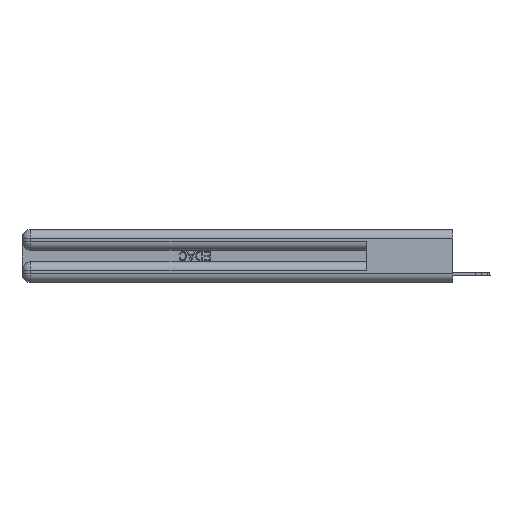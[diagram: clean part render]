
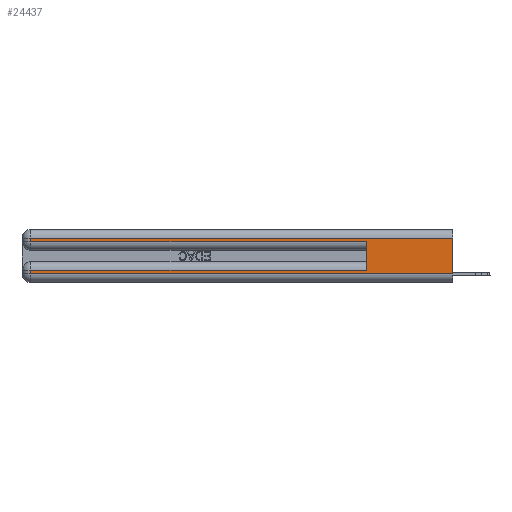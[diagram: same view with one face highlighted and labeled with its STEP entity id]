
A CAD part, left-side view. The second image highlights one B-rep face of the part: STEP entity #24437.
In plain terms, the highlighted planar face has unit normal (-1, 0, 0).
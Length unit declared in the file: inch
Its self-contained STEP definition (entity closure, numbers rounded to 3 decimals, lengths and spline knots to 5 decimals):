
#738 = EDGE_CURVE ( 'NONE', #1141, #9404, #14816, .T. ) ;
#751 = DIRECTION ( 'NONE',  ( 0., 0., -1. ) ) ;
#999 = LINE ( 'NONE', #17938, #28535 ) ;
#1023 = ORIENTED_EDGE ( 'NONE', *, *, #23884, .T. ) ;
#1141 = VERTEX_POINT ( 'NONE', #7086 ) ;
#3036 = LINE ( 'NONE', #12337, #10934 ) ;
#3364 = VECTOR ( 'NONE', #19117, 39.37008 ) ;
#3694 = ORIENTED_EDGE ( 'NONE', *, *, #4199, .T. ) ;
#4199 = EDGE_CURVE ( 'NONE', #7396, #12681, #21304, .T. ) ;
#4315 = VERTEX_POINT ( 'NONE', #29066 ) ;
#4872 = PLANE ( 'NONE',  #8600 ) ;
#5170 = VECTOR ( 'NONE', #24261, 39.37008 ) ;
#5258 = DIRECTION ( 'NONE',  ( 0., 1., 0. ) ) ;
#5300 = DIRECTION ( 'NONE',  ( 0., -1., 0. ) ) ;
#5316 = DIRECTION ( 'NONE',  ( 0., 0., -1. ) ) ;
#5409 = CARTESIAN_POINT ( 'NONE',  ( 0., 0., 0.085 ) ) ;
#6192 = EDGE_CURVE ( 'NONE', #12681, #4315, #3036, .T. ) ;
#7086 = CARTESIAN_POINT ( 'NONE',  ( 0., 0., 0.31 ) ) ;
#7396 = VERTEX_POINT ( 'NONE', #23852 ) ;
#8534 = VECTOR ( 'NONE', #5300, 39.37008 ) ;
#8600 = AXIS2_PLACEMENT_3D ( 'NONE', #16933, #12188, #5316 ) ;
#8640 = DIRECTION ( 'NONE',  ( 0., -1., 0. ) ) ;
#9404 = VERTEX_POINT ( 'NONE', #16641 ) ;
#9661 = VERTEX_POINT ( 'NONE', #19988 ) ;
#9787 = CARTESIAN_POINT ( 'NONE',  ( 0., 0., 0.37 ) ) ;
#10868 = EDGE_CURVE ( 'NONE', #7396, #14240, #19543, .T. ) ;
#10934 = VECTOR ( 'NONE', #751, 39.37008 ) ;
#12188 = DIRECTION ( 'NONE',  ( 1., 0., 0. ) ) ;
#12332 = CARTESIAN_POINT ( 'NONE',  ( 0., 0.6, 0.145 ) ) ;
#12337 = CARTESIAN_POINT ( 'NONE',  ( 0., 2.94, 0.37 ) ) ;
#12482 = FACE_OUTER_BOUND ( 'NONE', #23124, .T. ) ;
#12681 = VERTEX_POINT ( 'NONE', #25289 ) ;
#13088 = ORIENTED_EDGE ( 'NONE', *, *, #10868, .F. ) ;
#13184 = DIRECTION ( 'NONE',  ( 0., 0., -1. ) ) ;
#14240 = VERTEX_POINT ( 'NONE', #28655 ) ;
#14816 = LINE ( 'NONE', #9787, #3364 ) ;
#14958 = ORIENTED_EDGE ( 'NONE', *, *, #29106, .T. ) ;
#15776 = LINE ( 'NONE', #29975, #22240 ) ;
#16052 = VECTOR ( 'NONE', #5258, 39.37008 ) ;
#16392 = CARTESIAN_POINT ( 'NONE',  ( 0., 0., 0.06 ) ) ;
#16641 = CARTESIAN_POINT ( 'NONE',  ( 0., 0., 0.06 ) ) ;
#16914 = LINE ( 'NONE', #26237, #8534 ) ;
#16933 = CARTESIAN_POINT ( 'NONE',  ( 0., 0., 0.37 ) ) ;
#17938 = CARTESIAN_POINT ( 'NONE',  ( 0., 2.94, 0.37 ) ) ;
#19117 = DIRECTION ( 'NONE',  ( 0., 0., -1. ) ) ;
#19303 = ORIENTED_EDGE ( 'NONE', *, *, #6192, .T. ) ;
#19543 = LINE ( 'NONE', #12332, #5170 ) ;
#19988 = CARTESIAN_POINT ( 'NONE',  ( 0., 2.94, 0.31 ) ) ;
#21304 = LINE ( 'NONE', #5409, #16052 ) ;
#22178 = EDGE_CURVE ( 'NONE', #4315, #9404, #29397, .T. ) ;
#22217 = VECTOR ( 'NONE', #8640, 39.37008 ) ;
#22240 = VECTOR ( 'NONE', #25269, 39.37008 ) ;
#23124 = EDGE_LOOP ( 'NONE', ( #28944, #1023, #24727, #14958, #13088, #3694, #19303, #23872 ) ) ;
#23642 = VERTEX_POINT ( 'NONE', #26811 ) ;
#23852 = CARTESIAN_POINT ( 'NONE',  ( 0., 0.6, 0.085 ) ) ;
#23872 = ORIENTED_EDGE ( 'NONE', *, *, #22178, .T. ) ;
#23884 = EDGE_CURVE ( 'NONE', #1141, #9661, #15776, .T. ) ;
#24261 = DIRECTION ( 'NONE',  ( 0., 0., 1. ) ) ;
#24437 = ADVANCED_FACE ( 'NONE', ( #12482 ), #4872, .F. ) ;
#24727 = ORIENTED_EDGE ( 'NONE', *, *, #29246, .T. ) ;
#25269 = DIRECTION ( 'NONE',  ( 0., 1., 0. ) ) ;
#25289 = CARTESIAN_POINT ( 'NONE',  ( 0., 2.94, 0.085 ) ) ;
#26237 = CARTESIAN_POINT ( 'NONE',  ( 0., 0., 0.285 ) ) ;
#26811 = CARTESIAN_POINT ( 'NONE',  ( 0., 2.94, 0.285 ) ) ;
#28535 = VECTOR ( 'NONE', #13184, 39.37008 ) ;
#28655 = CARTESIAN_POINT ( 'NONE',  ( 0., 0.6, 0.285 ) ) ;
#28944 = ORIENTED_EDGE ( 'NONE', *, *, #738, .F. ) ;
#29066 = CARTESIAN_POINT ( 'NONE',  ( 0., 2.94, 0.06 ) ) ;
#29106 = EDGE_CURVE ( 'NONE', #23642, #14240, #16914, .T. ) ;
#29246 = EDGE_CURVE ( 'NONE', #9661, #23642, #999, .T. ) ;
#29397 = LINE ( 'NONE', #16392, #22217 ) ;
#29975 = CARTESIAN_POINT ( 'NONE',  ( 0., 0., 0.31 ) ) ;
